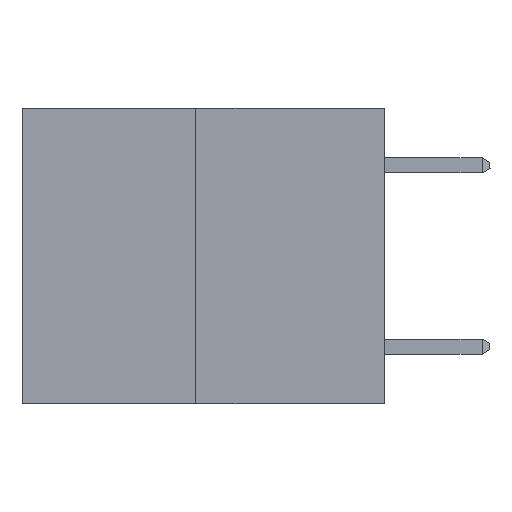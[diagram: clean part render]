
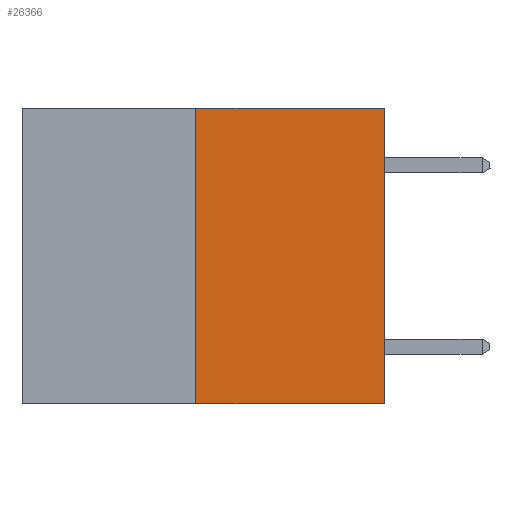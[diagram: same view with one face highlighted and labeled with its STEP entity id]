
A CAD part, left-side view. The second image highlights one B-rep face of the part: STEP entity #26366.
In plain terms, the highlighted planar face has unit normal (-1, 0, 0).
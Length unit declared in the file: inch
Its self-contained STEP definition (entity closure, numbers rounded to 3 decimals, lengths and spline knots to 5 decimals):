
#371 = VECTOR ( 'NONE', #23188, 39.37008 ) ;
#502 = CARTESIAN_POINT ( 'NONE',  ( 0., 0.312, -0.49 ) ) ;
#659 = EDGE_CURVE ( 'NONE', #13335, #22395, #28079, .T. ) ;
#1445 = EDGE_CURVE ( 'NONE', #13335, #17847, #13221, .T. ) ;
#1595 = ORIENTED_EDGE ( 'NONE', *, *, #659, .F. ) ;
#3856 = ORIENTED_EDGE ( 'NONE', *, *, #1445, .T. ) ;
#4963 = CARTESIAN_POINT ( 'NONE',  ( 0., 0.312, -0.49 ) ) ;
#6771 = CARTESIAN_POINT ( 'NONE',  ( 0., 0.6, 0. ) ) ;
#9554 = DIRECTION ( 'NONE',  ( 0., 0., 1. ) ) ;
#12619 = AXIS2_PLACEMENT_3D ( 'NONE', #16828, #31131, #14286 ) ;
#12700 = EDGE_CURVE ( 'NONE', #17847, #20500, #25010, .T. ) ;
#13221 = LINE ( 'NONE', #25929, #371 ) ;
#13335 = VERTEX_POINT ( 'NONE', #4963 ) ;
#13829 = ORIENTED_EDGE ( 'NONE', *, *, #20142, .F. ) ;
#13881 = CARTESIAN_POINT ( 'NONE',  ( 0., 0.312, 0. ) ) ;
#14286 = DIRECTION ( 'NONE',  ( 0., 0., -1. ) ) ;
#14454 = FACE_OUTER_BOUND ( 'NONE', #21359, .T. ) ;
#16828 = CARTESIAN_POINT ( 'NONE',  ( 0., 0.6, 0. ) ) ;
#17847 = VERTEX_POINT ( 'NONE', #25663 ) ;
#20142 = EDGE_CURVE ( 'NONE', #22395, #20500, #21784, .T. ) ;
#20500 = VERTEX_POINT ( 'NONE', #30660 ) ;
#21359 = EDGE_LOOP ( 'NONE', ( #1595, #3856, #31164, #13829 ) ) ;
#21640 = VECTOR ( 'NONE', #27606, 39.37008 ) ;
#21717 = CARTESIAN_POINT ( 'NONE',  ( 0., 0., 0. ) ) ;
#21784 = LINE ( 'NONE', #6771, #29361 ) ;
#22395 = VERTEX_POINT ( 'NONE', #13881 ) ;
#23188 = DIRECTION ( 'NONE',  ( 0., -1., 0. ) ) ;
#24626 = VECTOR ( 'NONE', #9554, 39.37008 ) ;
#25010 = LINE ( 'NONE', #21717, #24626 ) ;
#25663 = CARTESIAN_POINT ( 'NONE',  ( 0., 0., -0.49 ) ) ;
#25929 = CARTESIAN_POINT ( 'NONE',  ( 0., 0.6, -0.49 ) ) ;
#26366 = ADVANCED_FACE ( 'NONE', ( #14454 ), #28817, .F. ) ;
#27606 = DIRECTION ( 'NONE',  ( 0., 0., 1. ) ) ;
#28079 = LINE ( 'NONE', #502, #21640 ) ;
#28469 = DIRECTION ( 'NONE',  ( 0., -1., 0. ) ) ;
#28817 = PLANE ( 'NONE',  #12619 ) ;
#29361 = VECTOR ( 'NONE', #28469, 39.37008 ) ;
#30660 = CARTESIAN_POINT ( 'NONE',  ( 0., 0., 0. ) ) ;
#31131 = DIRECTION ( 'NONE',  ( 1., 0., 0. ) ) ;
#31164 = ORIENTED_EDGE ( 'NONE', *, *, #12700, .T. ) ;
